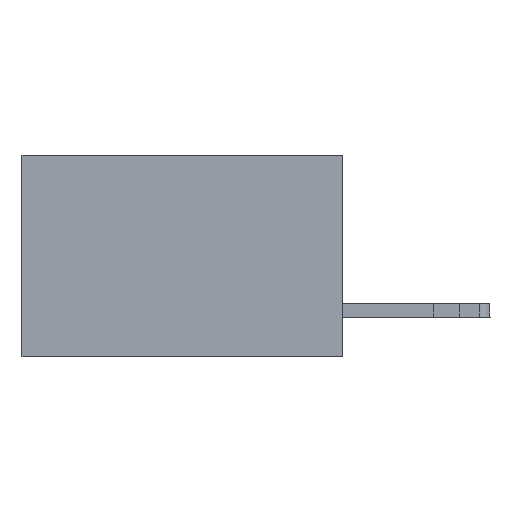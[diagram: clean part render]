
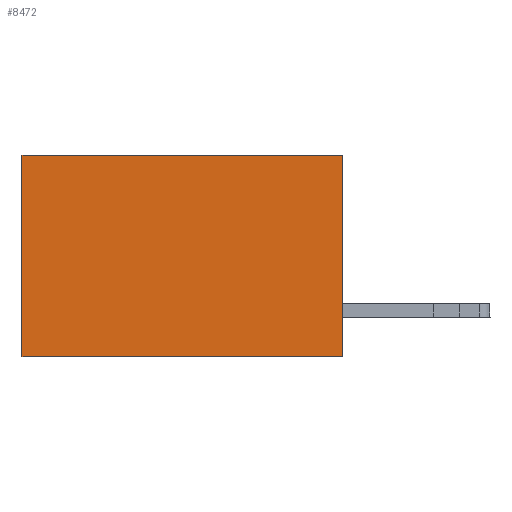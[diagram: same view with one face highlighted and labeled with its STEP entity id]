
A CAD part, left-side view. The second image highlights one B-rep face of the part: STEP entity #8472.
In plain terms, the highlighted planar face has unit normal (-1, 0, 0).
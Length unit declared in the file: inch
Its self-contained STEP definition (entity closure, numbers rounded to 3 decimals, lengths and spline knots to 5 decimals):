
#587 = CARTESIAN_POINT ( 'NONE',  ( 0.277, 0., 0. ) ) ;
#1516 = CARTESIAN_POINT ( 'NONE',  ( 0.277, 0., -0.37 ) ) ;
#2088 = EDGE_CURVE ( 'NONE', #11229, #3581, #24304, .T. ) ;
#2101 = CARTESIAN_POINT ( 'NONE',  ( 0.277, 0., 0. ) ) ;
#2344 = CARTESIAN_POINT ( 'NONE',  ( 0.277, 0., -0.37 ) ) ;
#2617 = VECTOR ( 'NONE', #17698, 39.37008 ) ;
#3581 = VERTEX_POINT ( 'NONE', #18232 ) ;
#4058 = VECTOR ( 'NONE', #18624, 39.37008 ) ;
#4559 = LINE ( 'NONE', #587, #8343 ) ;
#6160 = CARTESIAN_POINT ( 'NONE',  ( 0.277, 0., -0.37 ) ) ;
#6325 = DIRECTION ( 'NONE',  ( 1., 0., 0. ) ) ;
#6986 = CARTESIAN_POINT ( 'NONE',  ( 0.277, 0.59, -0.37 ) ) ;
#7226 = EDGE_CURVE ( 'NONE', #9722, #17376, #4559, .T. ) ;
#7998 = ORIENTED_EDGE ( 'NONE', *, *, #7226, .T. ) ;
#8343 = VECTOR ( 'NONE', #16614, 39.37008 ) ;
#8450 = FACE_OUTER_BOUND ( 'NONE', #19913, .T. ) ;
#8472 = ADVANCED_FACE ( 'NONE', ( #8450 ), #24459, .F. ) ;
#9722 = VERTEX_POINT ( 'NONE', #2101 ) ;
#10069 = AXIS2_PLACEMENT_3D ( 'NONE', #2344, #6325, #18504 ) ;
#10167 = EDGE_CURVE ( 'NONE', #9722, #11229, #22181, .T. ) ;
#11229 = VERTEX_POINT ( 'NONE', #1516 ) ;
#13037 = VECTOR ( 'NONE', #24431, 39.37008 ) ;
#13306 = ORIENTED_EDGE ( 'NONE', *, *, #2088, .F. ) ;
#14495 = CARTESIAN_POINT ( 'NONE',  ( 0.277, 0.59, 0. ) ) ;
#16614 = DIRECTION ( 'NONE',  ( 0., 1., 0. ) ) ;
#17054 = LINE ( 'NONE', #6986, #2617 ) ;
#17376 = VERTEX_POINT ( 'NONE', #14495 ) ;
#17698 = DIRECTION ( 'NONE',  ( 0., 0., -1. ) ) ;
#18232 = CARTESIAN_POINT ( 'NONE',  ( 0.277, 0.59, -0.37 ) ) ;
#18454 = EDGE_CURVE ( 'NONE', #17376, #3581, #17054, .T. ) ;
#18504 = DIRECTION ( 'NONE',  ( 0., 0., -1. ) ) ;
#18624 = DIRECTION ( 'NONE',  ( 0., 1., 0. ) ) ;
#19626 = ORIENTED_EDGE ( 'NONE', *, *, #10167, .F. ) ;
#19913 = EDGE_LOOP ( 'NONE', ( #23719, #13306, #19626, #7998 ) ) ;
#22181 = LINE ( 'NONE', #6160, #13037 ) ;
#22321 = CARTESIAN_POINT ( 'NONE',  ( 0.277, 0., -0.37 ) ) ;
#23719 = ORIENTED_EDGE ( 'NONE', *, *, #18454, .T. ) ;
#24304 = LINE ( 'NONE', #22321, #4058 ) ;
#24431 = DIRECTION ( 'NONE',  ( 0., 0., -1. ) ) ;
#24459 = PLANE ( 'NONE',  #10069 ) ;
